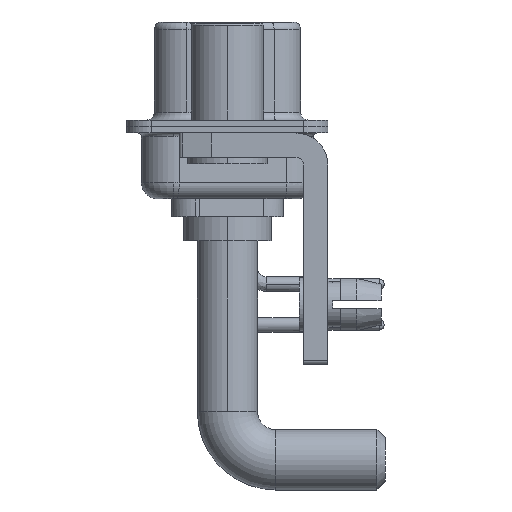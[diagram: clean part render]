
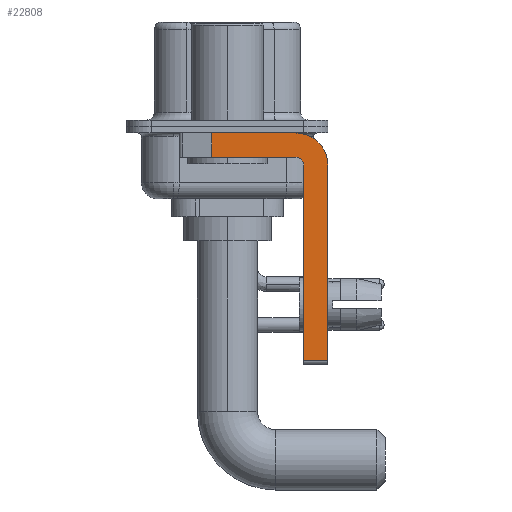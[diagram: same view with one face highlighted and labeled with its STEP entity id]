
A CAD part, left-side view. The second image highlights one B-rep face of the part: STEP entity #22808.
In plain terms, the highlighted planar face has unit normal (-1, 0, 0).
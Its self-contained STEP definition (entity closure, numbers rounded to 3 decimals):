
#448 = VERTEX_POINT ( 'NONE', #24513 ) ;
#483 = VERTEX_POINT ( 'NONE', #30112 ) ;
#763 = CARTESIAN_POINT ( 'NONE',  ( -2.9, -6.25, -14.55 ) ) ;
#971 = ORIENTED_EDGE ( 'NONE', *, *, #19231, .F. ) ;
#1046 = DIRECTION ( 'NONE',  ( 0., 0., -1. ) ) ;
#1539 = CARTESIAN_POINT ( 'NONE',  ( -2.9, -4.25, -2.4 ) ) ;
#2483 = VERTEX_POINT ( 'NONE', #17698 ) ;
#2773 = CARTESIAN_POINT ( 'NONE',  ( -2.9, 0.978, -1.9 ) ) ;
#2946 = EDGE_CURVE ( 'NONE', #4517, #4159, #13358, .T. ) ;
#2982 = LINE ( 'NONE', #22197, #23313 ) ;
#3729 = ORIENTED_EDGE ( 'NONE', *, *, #25156, .F. ) ;
#4015 = PLANE ( 'NONE',  #22646 ) ;
#4159 = VERTEX_POINT ( 'NONE', #2773 ) ;
#4216 = DIRECTION ( 'NONE',  ( -1., 0., 0. ) ) ;
#4397 = EDGE_CURVE ( 'NONE', #22155, #2483, #4702, .T. ) ;
#4517 = VERTEX_POINT ( 'NONE', #26004 ) ;
#4702 = LINE ( 'NONE', #5018, #23576 ) ;
#5018 = CARTESIAN_POINT ( 'NONE',  ( -2.9, 3., -0.4 ) ) ;
#5081 = ORIENTED_EDGE ( 'NONE', *, *, #15317, .F. ) ;
#5439 = VECTOR ( 'NONE', #7575, 1000. ) ;
#5524 = ORIENTED_EDGE ( 'NONE', *, *, #2946, .F. ) ;
#6183 = CARTESIAN_POINT ( 'NONE',  ( -2.9, -6.25, -2.4 ) ) ;
#7575 = DIRECTION ( 'NONE',  ( 0., -1., 0. ) ) ;
#7727 = CARTESIAN_POINT ( 'NONE',  ( -2.9, -4.25, -14.55 ) ) ;
#8043 = EDGE_CURVE ( 'NONE', #448, #24116, #30359, .T. ) ;
#8868 = EDGE_LOOP ( 'NONE', ( #9127, #31965, #5524, #5081, #3729, #12853, #19029, #971 ) ) ;
#9015 = DIRECTION ( 'NONE',  ( 0., 0., 1. ) ) ;
#9127 = ORIENTED_EDGE ( 'NONE', *, *, #4397, .F. ) ;
#12165 = CARTESIAN_POINT ( 'NONE',  ( -2.9, -6.25, -2.4 ) ) ;
#12853 = ORIENTED_EDGE ( 'NONE', *, *, #8043, .T. ) ;
#13358 = LINE ( 'NONE', #31528, #26218 ) ;
#14376 = DIRECTION ( 'NONE',  ( 0., 0., -1. ) ) ;
#14991 = VERTEX_POINT ( 'NONE', #12165 ) ;
#15166 = VECTOR ( 'NONE', #1046, 1000. ) ;
#15317 = EDGE_CURVE ( 'NONE', #483, #4517, #29362, .T. ) ;
#16790 = CARTESIAN_POINT ( 'NONE',  ( -2.9, -4.25, -2.4 ) ) ;
#17280 = CIRCLE ( 'NONE', #21517, 2. ) ;
#17698 = CARTESIAN_POINT ( 'NONE',  ( -2.9, -4.25, -0.4 ) ) ;
#19029 = ORIENTED_EDGE ( 'NONE', *, *, #21351, .F. ) ;
#19231 = EDGE_CURVE ( 'NONE', #2483, #14991, #17280, .T. ) ;
#19857 = CARTESIAN_POINT ( 'NONE',  ( -2.9, -4.25, -2.4 ) ) ;
#20878 = DIRECTION ( 'NONE',  ( 1., 0., 0. ) ) ;
#21351 = EDGE_CURVE ( 'NONE', #14991, #24116, #23681, .T. ) ;
#21517 = AXIS2_PLACEMENT_3D ( 'NONE', #19857, #27757, #27930 ) ;
#22155 = VERTEX_POINT ( 'NONE', #29882 ) ;
#22197 = CARTESIAN_POINT ( 'NONE',  ( -2.9, -4.75, -14.8 ) ) ;
#22646 = AXIS2_PLACEMENT_3D ( 'NONE', #1539, #20878, #30955 ) ;
#22679 = DIRECTION ( 'NONE',  ( 0., -1., 0. ) ) ;
#22808 = ADVANCED_FACE ( 'NONE', ( #26179 ), #4015, .F. ) ;
#23313 = VECTOR ( 'NONE', #25620, 1000. ) ;
#23395 = EDGE_CURVE ( 'NONE', #22155, #4159, #29729, .T. ) ;
#23576 = VECTOR ( 'NONE', #22679, 1000. ) ;
#23681 = LINE ( 'NONE', #6183, #15166 ) ;
#23919 = DIRECTION ( 'NONE',  ( 0., 1., 0. ) ) ;
#24116 = VERTEX_POINT ( 'NONE', #763 ) ;
#24130 = CARTESIAN_POINT ( 'NONE',  ( -2.9, 0.978, -1.9 ) ) ;
#24513 = CARTESIAN_POINT ( 'NONE',  ( -2.9, -4.75, -14.55 ) ) ;
#24622 = AXIS2_PLACEMENT_3D ( 'NONE', #16790, #4216, #9015 ) ;
#25156 = EDGE_CURVE ( 'NONE', #448, #483, #2982, .T. ) ;
#25620 = DIRECTION ( 'NONE',  ( 0., 0., 1. ) ) ;
#26004 = CARTESIAN_POINT ( 'NONE',  ( -2.9, -4.25, -1.9 ) ) ;
#26179 = FACE_OUTER_BOUND ( 'NONE', #8868, .T. ) ;
#26218 = VECTOR ( 'NONE', #23919, 1000. ) ;
#26375 = VECTOR ( 'NONE', #14376, 1000. ) ;
#27757 = DIRECTION ( 'NONE',  ( 1., 0., 0. ) ) ;
#27930 = DIRECTION ( 'NONE',  ( 0., 0., -1. ) ) ;
#29362 = CIRCLE ( 'NONE', #24622, 0.5 ) ;
#29729 = LINE ( 'NONE', #24130, #26375 ) ;
#29882 = CARTESIAN_POINT ( 'NONE',  ( -2.9, 0.978, -0.4 ) ) ;
#30112 = CARTESIAN_POINT ( 'NONE',  ( -2.9, -4.75, -2.4 ) ) ;
#30359 = LINE ( 'NONE', #7727, #5439 ) ;
#30955 = DIRECTION ( 'NONE',  ( 0., 0., -1. ) ) ;
#31528 = CARTESIAN_POINT ( 'NONE',  ( -2.9, -4.25, -1.9 ) ) ;
#31965 = ORIENTED_EDGE ( 'NONE', *, *, #23395, .T. ) ;
